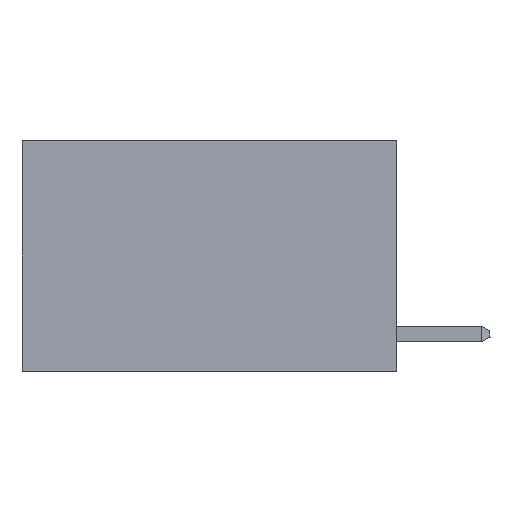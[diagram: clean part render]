
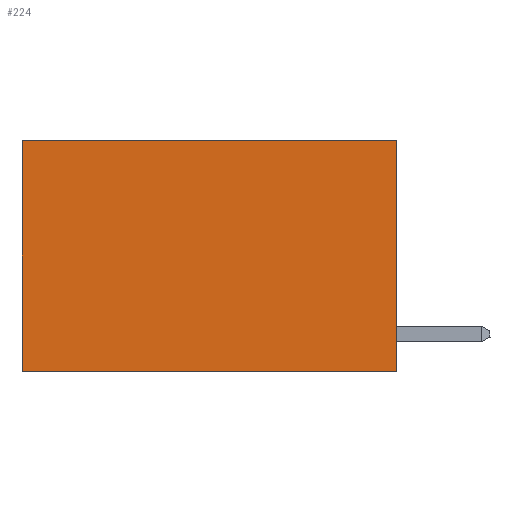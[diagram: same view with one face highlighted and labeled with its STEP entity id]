
A CAD part, left-side view. The second image highlights one B-rep face of the part: STEP entity #224.
In plain terms, the highlighted planar face has unit normal (-1, 0, 0).
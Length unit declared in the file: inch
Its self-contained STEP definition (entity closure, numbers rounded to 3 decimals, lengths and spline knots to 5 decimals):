
#77 = EDGE_CURVE ( 'NONE', #882, #2561, #6461, .T. ) ;
#97 = DIRECTION ( 'NONE',  ( 0., 1., 0. ) ) ;
#224 = ADVANCED_FACE ( 'NONE', ( #1012 ), #5476, .F. ) ;
#458 = LINE ( 'NONE', #2782, #5203 ) ;
#801 = VECTOR ( 'NONE', #97, 39.37008 ) ;
#882 = VERTEX_POINT ( 'NONE', #10595 ) ;
#978 = LINE ( 'NONE', #3691, #11037 ) ;
#1012 = FACE_OUTER_BOUND ( 'NONE', #6489, .T. ) ;
#1159 = VERTEX_POINT ( 'NONE', #6716 ) ;
#1891 = EDGE_CURVE ( 'NONE', #882, #4567, #978, .T. ) ;
#2561 = VERTEX_POINT ( 'NONE', #4151 ) ;
#2782 = CARTESIAN_POINT ( 'NONE',  ( 0.2625, 0.6, 0. ) ) ;
#3691 = CARTESIAN_POINT ( 'NONE',  ( 0.2625, 0., 0. ) ) ;
#4151 = CARTESIAN_POINT ( 'NONE',  ( 0.2625, 0.6, 0. ) ) ;
#4189 = AXIS2_PLACEMENT_3D ( 'NONE', #5544, #8799, #11595 ) ;
#4567 = VERTEX_POINT ( 'NONE', #10891 ) ;
#5203 = VECTOR ( 'NONE', #10482, 39.37008 ) ;
#5246 = EDGE_CURVE ( 'NONE', #4567, #1159, #8342, .T. ) ;
#5476 = PLANE ( 'NONE',  #4189 ) ;
#5544 = CARTESIAN_POINT ( 'NONE',  ( 0.2625, 0., 0. ) ) ;
#6266 = EDGE_CURVE ( 'NONE', #2561, #1159, #458, .T. ) ;
#6391 = ORIENTED_EDGE ( 'NONE', *, *, #77, .T. ) ;
#6461 = LINE ( 'NONE', #9263, #11220 ) ;
#6489 = EDGE_LOOP ( 'NONE', ( #7904, #11553, #10304, #6391 ) ) ;
#6716 = CARTESIAN_POINT ( 'NONE',  ( 0.2625, 0.6, -0.37 ) ) ;
#7904 = ORIENTED_EDGE ( 'NONE', *, *, #6266, .T. ) ;
#8043 = CARTESIAN_POINT ( 'NONE',  ( 0.2625, 0., -0.37 ) ) ;
#8342 = LINE ( 'NONE', #8043, #801 ) ;
#8799 = DIRECTION ( 'NONE',  ( 1., 0., 0. ) ) ;
#9263 = CARTESIAN_POINT ( 'NONE',  ( 0.2625, 0., 0. ) ) ;
#9289 = DIRECTION ( 'NONE',  ( 0., 1., 0. ) ) ;
#10304 = ORIENTED_EDGE ( 'NONE', *, *, #1891, .F. ) ;
#10482 = DIRECTION ( 'NONE',  ( 0., 0., -1. ) ) ;
#10595 = CARTESIAN_POINT ( 'NONE',  ( 0.2625, 0., 0. ) ) ;
#10891 = CARTESIAN_POINT ( 'NONE',  ( 0.2625, 0., -0.37 ) ) ;
#11037 = VECTOR ( 'NONE', #11351, 39.37008 ) ;
#11220 = VECTOR ( 'NONE', #9289, 39.37008 ) ;
#11351 = DIRECTION ( 'NONE',  ( 0., 0., -1. ) ) ;
#11553 = ORIENTED_EDGE ( 'NONE', *, *, #5246, .F. ) ;
#11595 = DIRECTION ( 'NONE',  ( 0., 0., -1. ) ) ;
